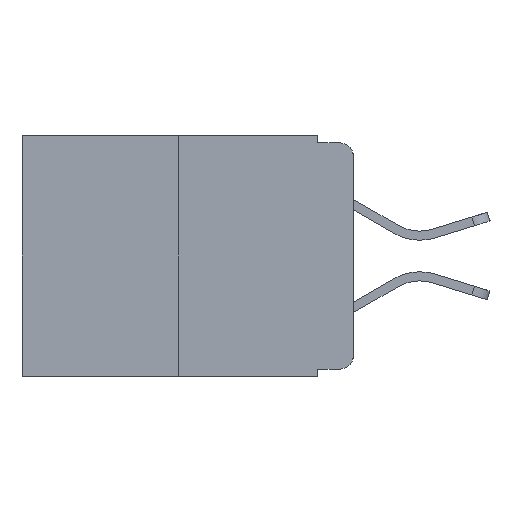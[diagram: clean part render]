
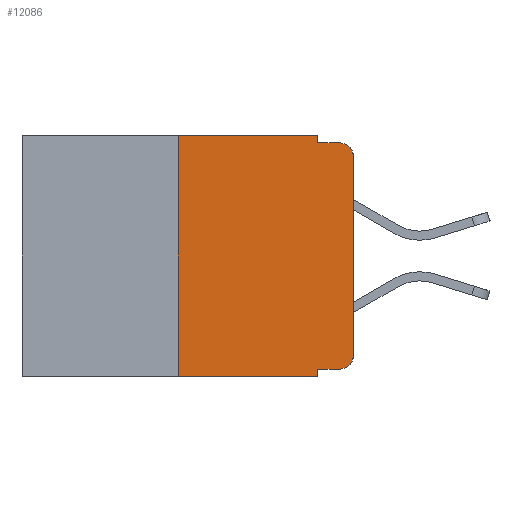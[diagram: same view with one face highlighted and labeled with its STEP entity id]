
A CAD part, left-side view. The second image highlights one B-rep face of the part: STEP entity #12086.
In plain terms, the highlighted planar face has unit normal (-1, 0, 0).
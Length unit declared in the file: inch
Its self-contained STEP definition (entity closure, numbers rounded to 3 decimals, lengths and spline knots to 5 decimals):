
#225 = ORIENTED_EDGE ( 'NONE', *, *, #11232, .F. ) ;
#475 = VERTEX_POINT ( 'NONE', #6734 ) ;
#630 = ORIENTED_EDGE ( 'NONE', *, *, #4097, .T. ) ;
#1091 = VECTOR ( 'NONE', #14723, 39.37008 ) ;
#1483 = LINE ( 'NONE', #23111, #18630 ) ;
#1560 = DIRECTION ( 'NONE',  ( 0., 0., -1. ) ) ;
#1667 = VECTOR ( 'NONE', #5804, 39.37008 ) ;
#1685 = DIRECTION ( 'NONE',  ( 1., 0., 0. ) ) ;
#1900 = ORIENTED_EDGE ( 'NONE', *, *, #3615, .F. ) ;
#2042 = CARTESIAN_POINT ( 'NONE',  ( 0., 0.25, 0. ) ) ;
#2050 = CIRCLE ( 'NONE', #5128, 0.02 ) ;
#2629 = DIRECTION ( 'NONE',  ( 0., -1., 0. ) ) ;
#3064 = AXIS2_PLACEMENT_3D ( 'NONE', #7269, #1685, #1560 ) ;
#3615 = EDGE_CURVE ( 'NONE', #21196, #7105, #7918, .T. ) ;
#3627 = PLANE ( 'NONE',  #3064 ) ;
#3725 = EDGE_CURVE ( 'NONE', #6459, #16492, #2050, .T. ) ;
#3869 = CARTESIAN_POINT ( 'NONE',  ( 0., 0.051, 0. ) ) ;
#4079 = EDGE_CURVE ( 'NONE', #18702, #4554, #17048, .T. ) ;
#4097 = EDGE_CURVE ( 'NONE', #13791, #475, #18888, .T. ) ;
#4554 = VERTEX_POINT ( 'NONE', #2042 ) ;
#4660 = EDGE_CURVE ( 'NONE', #17087, #475, #1483, .T. ) ;
#4831 = VECTOR ( 'NONE', #19009, 39.37008 ) ;
#5128 = AXIS2_PLACEMENT_3D ( 'NONE', #21346, #6925, #12308 ) ;
#5456 = LINE ( 'NONE', #13022, #1667 ) ;
#5804 = DIRECTION ( 'NONE',  ( 0., 0., -1. ) ) ;
#5943 = DIRECTION ( 'NONE',  ( 0., 0., -1. ) ) ;
#6063 = DIRECTION ( 'NONE',  ( -1., 0., 0. ) ) ;
#6459 = VERTEX_POINT ( 'NONE', #21982 ) ;
#6734 = CARTESIAN_POINT ( 'NONE',  ( 0., 0.02, -0.01 ) ) ;
#6794 = DIRECTION ( 'NONE',  ( 0., -1., 0. ) ) ;
#6895 = EDGE_LOOP ( 'NONE', ( #21776, #630, #19235, #16255, #225, #17209, #12261, #1900, #10400, #13143 ) ) ;
#6925 = DIRECTION ( 'NONE',  ( -1., 0., 0. ) ) ;
#6994 = CARTESIAN_POINT ( 'NONE',  ( 0., 0., -0.03 ) ) ;
#7105 = VERTEX_POINT ( 'NONE', #15675 ) ;
#7144 = CARTESIAN_POINT ( 'NONE',  ( 0., 0.051, -0.333 ) ) ;
#7269 = CARTESIAN_POINT ( 'NONE',  ( 0., 0.473, 0. ) ) ;
#7918 = LINE ( 'NONE', #17077, #14918 ) ;
#7951 = DIRECTION ( 'NONE',  ( 0., 0., 1. ) ) ;
#10400 = ORIENTED_EDGE ( 'NONE', *, *, #11188, .T. ) ;
#10427 = EDGE_CURVE ( 'NONE', #16492, #13791, #15059, .T. ) ;
#10586 = LINE ( 'NONE', #21936, #12063 ) ;
#11081 = AXIS2_PLACEMENT_3D ( 'NONE', #18899, #6063, #5943 ) ;
#11188 = EDGE_CURVE ( 'NONE', #21196, #6459, #18246, .T. ) ;
#11232 = EDGE_CURVE ( 'NONE', #4554, #19018, #22992, .T. ) ;
#12063 = VECTOR ( 'NONE', #6794, 39.37008 ) ;
#12086 = ADVANCED_FACE ( 'NONE', ( #14358 ), #3627, .F. ) ;
#12261 = ORIENTED_EDGE ( 'NONE', *, *, #20165, .T. ) ;
#12308 = DIRECTION ( 'NONE',  ( 0., 0., -1. ) ) ;
#12357 = VECTOR ( 'NONE', #7951, 39.37008 ) ;
#13022 = CARTESIAN_POINT ( 'NONE',  ( 0., 0.051, 0. ) ) ;
#13097 = CARTESIAN_POINT ( 'NONE',  ( 0., 0., 0. ) ) ;
#13143 = ORIENTED_EDGE ( 'NONE', *, *, #3725, .T. ) ;
#13791 = VERTEX_POINT ( 'NONE', #6994 ) ;
#14358 = FACE_OUTER_BOUND ( 'NONE', #6895, .T. ) ;
#14723 = DIRECTION ( 'NONE',  ( 0., -1., 0. ) ) ;
#14918 = VECTOR ( 'NONE', #19390, 39.37008 ) ;
#15059 = LINE ( 'NONE', #13097, #12357 ) ;
#15675 = CARTESIAN_POINT ( 'NONE',  ( 0., 0.051, -0.343 ) ) ;
#15831 = CARTESIAN_POINT ( 'NONE',  ( 0., 0.25, -0.343 ) ) ;
#16255 = ORIENTED_EDGE ( 'NONE', *, *, #17645, .F. ) ;
#16275 = VECTOR ( 'NONE', #2629, 39.37008 ) ;
#16492 = VERTEX_POINT ( 'NONE', #17582 ) ;
#17048 = LINE ( 'NONE', #22790, #4831 ) ;
#17077 = CARTESIAN_POINT ( 'NONE',  ( 0., 0.051, 0. ) ) ;
#17087 = VERTEX_POINT ( 'NONE', #19761 ) ;
#17209 = ORIENTED_EDGE ( 'NONE', *, *, #4079, .F. ) ;
#17582 = CARTESIAN_POINT ( 'NONE',  ( 0., 0., -0.313 ) ) ;
#17645 = EDGE_CURVE ( 'NONE', #19018, #17087, #5456, .T. ) ;
#18246 = LINE ( 'NONE', #7144, #1091 ) ;
#18630 = VECTOR ( 'NONE', #21724, 39.37008 ) ;
#18702 = VERTEX_POINT ( 'NONE', #15831 ) ;
#18888 = CIRCLE ( 'NONE', #11081, 0.02 ) ;
#18899 = CARTESIAN_POINT ( 'NONE',  ( 0., 0.02, -0.03 ) ) ;
#19009 = DIRECTION ( 'NONE',  ( 0., 0., 1. ) ) ;
#19018 = VERTEX_POINT ( 'NONE', #3869 ) ;
#19235 = ORIENTED_EDGE ( 'NONE', *, *, #4660, .F. ) ;
#19390 = DIRECTION ( 'NONE',  ( 0., 0., -1. ) ) ;
#19761 = CARTESIAN_POINT ( 'NONE',  ( 0., 0.051, -0.01 ) ) ;
#20165 = EDGE_CURVE ( 'NONE', #18702, #7105, #10586, .T. ) ;
#21196 = VERTEX_POINT ( 'NONE', #23365 ) ;
#21346 = CARTESIAN_POINT ( 'NONE',  ( 0., 0.02, -0.313 ) ) ;
#21724 = DIRECTION ( 'NONE',  ( 0., -1., 0. ) ) ;
#21776 = ORIENTED_EDGE ( 'NONE', *, *, #10427, .T. ) ;
#21936 = CARTESIAN_POINT ( 'NONE',  ( 0., 0.473, -0.343 ) ) ;
#21982 = CARTESIAN_POINT ( 'NONE',  ( 0., 0.02, -0.333 ) ) ;
#22771 = CARTESIAN_POINT ( 'NONE',  ( 0., 0.473, 0. ) ) ;
#22790 = CARTESIAN_POINT ( 'NONE',  ( 0., 0.25, 0. ) ) ;
#22992 = LINE ( 'NONE', #22771, #16275 ) ;
#23111 = CARTESIAN_POINT ( 'NONE',  ( 0., 0.051, -0.01 ) ) ;
#23365 = CARTESIAN_POINT ( 'NONE',  ( 0., 0.051, -0.333 ) ) ;
